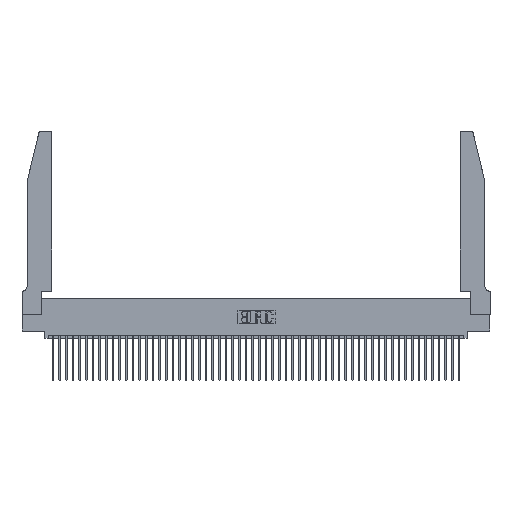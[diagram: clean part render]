
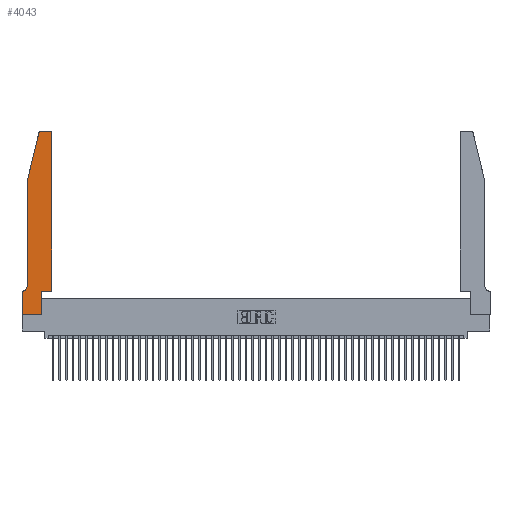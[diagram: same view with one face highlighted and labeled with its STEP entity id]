
A CAD part, top view. The second image highlights one B-rep face of the part: STEP entity #4043.
In plain terms, the highlighted planar face has unit normal (0, 0, 1).
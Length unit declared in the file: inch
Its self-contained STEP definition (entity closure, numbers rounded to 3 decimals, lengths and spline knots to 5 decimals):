
#420 = CIRCLE ( 'NONE', #11040, 0.03 ) ;
#2286 = ORIENTED_EDGE ( 'NONE', *, *, #20159, .T. ) ;
#2296 = DIRECTION ( 'NONE',  ( -1., 0., 0. ) ) ;
#2361 = DIRECTION ( 'NONE',  ( 1., 0., 0. ) ) ;
#2737 = DIRECTION ( 'NONE',  ( 0., -1., 0. ) ) ;
#3569 = CARTESIAN_POINT ( 'NONE',  ( 0.4505, 0.35, 0.37 ) ) ;
#3686 = EDGE_CURVE ( 'NONE', #30211, #5549, #42943, .T. ) ;
#4043 = ADVANCED_FACE ( 'NONE', ( #26950 ), #35567, .T. ) ;
#4086 = CARTESIAN_POINT ( 'NONE',  ( 0.2605, 2.75, 0.37 ) ) ;
#4160 = VECTOR ( 'NONE', #2296, 39.37008 ) ;
#5041 = CARTESIAN_POINT ( 'NONE',  ( 0.0755, 2., 0.37 ) ) ;
#5296 = CARTESIAN_POINT ( 'NONE',  ( 0., 0., 0.37 ) ) ;
#5549 = VERTEX_POINT ( 'NONE', #45072 ) ;
#6262 = VERTEX_POINT ( 'NONE', #5041 ) ;
#7336 = VERTEX_POINT ( 'NONE', #47034 ) ;
#8980 = CARTESIAN_POINT ( 'NONE',  ( 0.4205, 2.72, 0.37 ) ) ;
#9151 = EDGE_CURVE ( 'NONE', #6262, #31644, #15886, .T. ) ;
#9721 = EDGE_LOOP ( 'NONE', ( #50790, #13763, #50351, #47171, #2286, #34417, #23635, #28207, #45682, #13493, #43569, #37923 ) ) ;
#10042 = LINE ( 'NONE', #4086, #50661 ) ;
#10610 = LINE ( 'NONE', #25047, #30336 ) ;
#11040 = AXIS2_PLACEMENT_3D ( 'NONE', #8980, #36507, #12933 ) ;
#11571 = VECTOR ( 'NONE', #18087, 39.37008 ) ;
#12014 = DIRECTION ( 'NONE',  ( 0., 0., 1. ) ) ;
#12594 = CIRCLE ( 'NONE', #45386, 0.07 ) ;
#12670 = VECTOR ( 'NONE', #40012, 39.37008 ) ;
#12933 = DIRECTION ( 'NONE',  ( 1., 0., 0. ) ) ;
#13336 = DIRECTION ( 'NONE',  ( 1., 0., 0. ) ) ;
#13393 = CARTESIAN_POINT ( 'NONE',  ( 0.25487, 2.72718, 0.37 ) ) ;
#13477 = CARTESIAN_POINT ( 'NONE',  ( 0., 0., 0.37 ) ) ;
#13493 = ORIENTED_EDGE ( 'NONE', *, *, #34775, .T. ) ;
#13763 = ORIENTED_EDGE ( 'NONE', *, *, #32901, .T. ) ;
#14468 = CARTESIAN_POINT ( 'NONE',  ( 0.4205, 2.75, 0.37 ) ) ;
#15049 = VERTEX_POINT ( 'NONE', #14468 ) ;
#15625 = EDGE_CURVE ( 'NONE', #31686, #41642, #35514, .T. ) ;
#15667 = DIRECTION ( 'NONE',  ( 0., 0., -1. ) ) ;
#15886 = LINE ( 'NONE', #26276, #26363 ) ;
#16486 = VECTOR ( 'NONE', #31371, 39.37008 ) ;
#17283 = EDGE_CURVE ( 'NONE', #40430, #15049, #420, .T. ) ;
#18053 = EDGE_CURVE ( 'NONE', #18533, #6262, #41513, .T. ) ;
#18087 = DIRECTION ( 'NONE',  ( 1., 0., 0. ) ) ;
#18533 = VERTEX_POINT ( 'NONE', #13393 ) ;
#18852 = VERTEX_POINT ( 'NONE', #34860 ) ;
#18970 = EDGE_CURVE ( 'NONE', #15049, #18852, #10042, .T. ) ;
#18975 = LINE ( 'NONE', #26503, #16486 ) ;
#19579 = CARTESIAN_POINT ( 'NONE',  ( 0.4505, 2.72, 0.37 ) ) ;
#19770 = CARTESIAN_POINT ( 'NONE',  ( 0., 0.35, 0.37 ) ) ;
#19898 = DIRECTION ( 'NONE',  ( -1., 0., 0. ) ) ;
#20159 = EDGE_CURVE ( 'NONE', #31644, #31686, #12594, .T. ) ;
#22041 = CARTESIAN_POINT ( 'NONE',  ( 0., 0., 0.37 ) ) ;
#23635 = ORIENTED_EDGE ( 'NONE', *, *, #45615, .T. ) ;
#23754 = CIRCLE ( 'NONE', #29617, 0.03 ) ;
#25047 = CARTESIAN_POINT ( 'NONE',  ( 0.4505, 0.35, 0.37 ) ) ;
#25824 = EDGE_CURVE ( 'NONE', #29866, #40430, #44056, .T. ) ;
#25907 = DIRECTION ( 'NONE',  ( 0., 0., 1. ) ) ;
#26276 = CARTESIAN_POINT ( 'NONE',  ( 0.0755, 2., 0.37 ) ) ;
#26363 = VECTOR ( 'NONE', #2737, 39.37008 ) ;
#26503 = CARTESIAN_POINT ( 'NONE',  ( 0.2865, 0.35, 0.37 ) ) ;
#26950 = FACE_OUTER_BOUND ( 'NONE', #9721, .T. ) ;
#28207 = ORIENTED_EDGE ( 'NONE', *, *, #3686, .T. ) ;
#29617 = AXIS2_PLACEMENT_3D ( 'NONE', #49444, #25907, #2361 ) ;
#29866 = VERTEX_POINT ( 'NONE', #3569 ) ;
#30211 = VERTEX_POINT ( 'NONE', #13477 ) ;
#30336 = VECTOR ( 'NONE', #13336, 39.37008 ) ;
#31206 = CARTESIAN_POINT ( 'NONE',  ( 0., 0.35, 0.37 ) ) ;
#31371 = DIRECTION ( 'NONE',  ( 0., 1., 0. ) ) ;
#31644 = VERTEX_POINT ( 'NONE', #42332 ) ;
#31686 = VERTEX_POINT ( 'NONE', #46440 ) ;
#32901 = EDGE_CURVE ( 'NONE', #18852, #18533, #23754, .T. ) ;
#34417 = ORIENTED_EDGE ( 'NONE', *, *, #15625, .T. ) ;
#34775 = EDGE_CURVE ( 'NONE', #7336, #29866, #10610, .T. ) ;
#34860 = CARTESIAN_POINT ( 'NONE',  ( 0.284, 2.75, 0.37 ) ) ;
#35514 = LINE ( 'NONE', #37670, #4160 ) ;
#35567 = PLANE ( 'NONE',  #39021 ) ;
#35675 = VECTOR ( 'NONE', #40723, 39.37008 ) ;
#36065 = CARTESIAN_POINT ( 'NONE',  ( 0.4505, 0.35, 0.37 ) ) ;
#36507 = DIRECTION ( 'NONE',  ( 0., 0., 1. ) ) ;
#36916 = LINE ( 'NONE', #5296, #35675 ) ;
#37670 = CARTESIAN_POINT ( 'NONE',  ( 0.0755, 0.35, 0.37 ) ) ;
#37923 = ORIENTED_EDGE ( 'NONE', *, *, #17283, .T. ) ;
#39021 = AXIS2_PLACEMENT_3D ( 'NONE', #19770, #12014, #39523 ) ;
#39202 = CARTESIAN_POINT ( 'NONE',  ( 0.0055, 0.42, 0.37 ) ) ;
#39523 = DIRECTION ( 'NONE',  ( 1., 0., 0. ) ) ;
#40012 = DIRECTION ( 'NONE',  ( 0., 1., 0. ) ) ;
#40430 = VERTEX_POINT ( 'NONE', #19579 ) ;
#40564 = DIRECTION ( 'NONE',  ( -0.239, -0.971, 0. ) ) ;
#40723 = DIRECTION ( 'NONE',  ( 0., -1., 0. ) ) ;
#41513 = LINE ( 'NONE', #44527, #48250 ) ;
#41642 = VERTEX_POINT ( 'NONE', #31206 ) ;
#41673 = EDGE_CURVE ( 'NONE', #5549, #7336, #18975, .T. ) ;
#42332 = CARTESIAN_POINT ( 'NONE',  ( 0.0755, 0.42, 0.37 ) ) ;
#42943 = LINE ( 'NONE', #22041, #11571 ) ;
#43163 = DIRECTION ( 'NONE',  ( -1., 0., 0. ) ) ;
#43569 = ORIENTED_EDGE ( 'NONE', *, *, #25824, .T. ) ;
#44056 = LINE ( 'NONE', #36065, #12670 ) ;
#44527 = CARTESIAN_POINT ( 'NONE',  ( 0.0755, 2., 0.37 ) ) ;
#45072 = CARTESIAN_POINT ( 'NONE',  ( 0.2865, 0., 0.37 ) ) ;
#45386 = AXIS2_PLACEMENT_3D ( 'NONE', #39202, #15667, #43163 ) ;
#45615 = EDGE_CURVE ( 'NONE', #41642, #30211, #36916, .T. ) ;
#45682 = ORIENTED_EDGE ( 'NONE', *, *, #41673, .T. ) ;
#46440 = CARTESIAN_POINT ( 'NONE',  ( 0.0055, 0.35, 0.37 ) ) ;
#47034 = CARTESIAN_POINT ( 'NONE',  ( 0.2865, 0.35, 0.37 ) ) ;
#47171 = ORIENTED_EDGE ( 'NONE', *, *, #9151, .T. ) ;
#48250 = VECTOR ( 'NONE', #40564, 39.37008 ) ;
#49444 = CARTESIAN_POINT ( 'NONE',  ( 0.284, 2.72, 0.37 ) ) ;
#50351 = ORIENTED_EDGE ( 'NONE', *, *, #18053, .T. ) ;
#50661 = VECTOR ( 'NONE', #19898, 39.37008 ) ;
#50790 = ORIENTED_EDGE ( 'NONE', *, *, #18970, .T. ) ;
